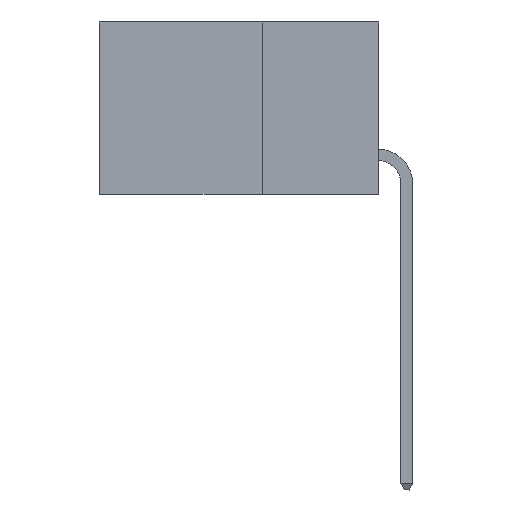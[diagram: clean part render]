
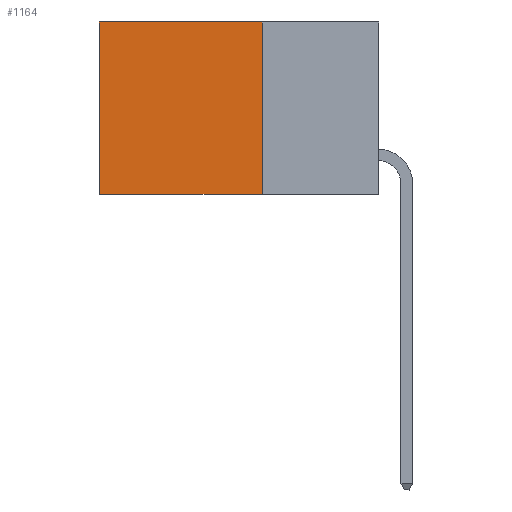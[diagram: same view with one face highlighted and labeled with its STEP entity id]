
A CAD part, left-side view. The second image highlights one B-rep face of the part: STEP entity #1164.
In plain terms, the highlighted planar face has unit normal (-1, 0, 0).
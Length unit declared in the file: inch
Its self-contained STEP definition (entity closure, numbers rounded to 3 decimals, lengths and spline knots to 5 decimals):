
#631 = VERTEX_POINT ( 'NONE', #17936 ) ;
#716 = LINE ( 'NONE', #8882, #4708 ) ;
#915 = VERTEX_POINT ( 'NONE', #16567 ) ;
#1164 = ADVANCED_FACE ( 'NONE', ( #8373 ), #3520, .F. ) ;
#2021 = VERTEX_POINT ( 'NONE', #2836 ) ;
#2396 = VECTOR ( 'NONE', #15899, 39.37008 ) ;
#2398 = VECTOR ( 'NONE', #8519, 39.37008 ) ;
#2538 = CARTESIAN_POINT ( 'NONE',  ( 0.2615, 0.25, 0. ) ) ;
#2836 = CARTESIAN_POINT ( 'NONE',  ( 0.2615, 0.25, 0. ) ) ;
#3272 = ORIENTED_EDGE ( 'NONE', *, *, #11680, .T. ) ;
#3520 = PLANE ( 'NONE',  #18665 ) ;
#3772 = EDGE_CURVE ( 'NONE', #2021, #915, #17835, .T. ) ;
#3941 = ORIENTED_EDGE ( 'NONE', *, *, #11051, .F. ) ;
#4708 = VECTOR ( 'NONE', #15148, 39.37008 ) ;
#6193 = EDGE_LOOP ( 'NONE', ( #3272, #3941, #19842, #14449 ) ) ;
#6678 = LINE ( 'NONE', #8411, #2396 ) ;
#6825 = DIRECTION ( 'NONE',  ( 1., 0., 0. ) ) ;
#8373 = FACE_OUTER_BOUND ( 'NONE', #6193, .T. ) ;
#8411 = CARTESIAN_POINT ( 'NONE',  ( 0.2615, 0.25, -0.37 ) ) ;
#8519 = DIRECTION ( 'NONE',  ( 0., 0., -1. ) ) ;
#8882 = CARTESIAN_POINT ( 'NONE',  ( 0.2615, 0.6, -0.37 ) ) ;
#8977 = VECTOR ( 'NONE', #17933, 39.37008 ) ;
#9718 = DIRECTION ( 'NONE',  ( 0., 0., -1. ) ) ;
#10059 = CARTESIAN_POINT ( 'NONE',  ( 0.2615, 0.25, -0.37 ) ) ;
#10268 = LINE ( 'NONE', #2538, #8977 ) ;
#11051 = EDGE_CURVE ( 'NONE', #915, #631, #6678, .T. ) ;
#11680 = EDGE_CURVE ( 'NONE', #17727, #631, #716, .T. ) ;
#14449 = ORIENTED_EDGE ( 'NONE', *, *, #16556, .T. ) ;
#14627 = CARTESIAN_POINT ( 'NONE',  ( 0.2615, 0.25, -0.37 ) ) ;
#14857 = CARTESIAN_POINT ( 'NONE',  ( 0.2615, 0.6, 0. ) ) ;
#15148 = DIRECTION ( 'NONE',  ( 0., 0., -1. ) ) ;
#15899 = DIRECTION ( 'NONE',  ( 0., 1., 0. ) ) ;
#16556 = EDGE_CURVE ( 'NONE', #2021, #17727, #10268, .T. ) ;
#16567 = CARTESIAN_POINT ( 'NONE',  ( 0.2615, 0.25, -0.37 ) ) ;
#17727 = VERTEX_POINT ( 'NONE', #14857 ) ;
#17835 = LINE ( 'NONE', #10059, #2398 ) ;
#17933 = DIRECTION ( 'NONE',  ( 0., 1., 0. ) ) ;
#17936 = CARTESIAN_POINT ( 'NONE',  ( 0.2615, 0.6, -0.37 ) ) ;
#18665 = AXIS2_PLACEMENT_3D ( 'NONE', #14627, #6825, #9718 ) ;
#19842 = ORIENTED_EDGE ( 'NONE', *, *, #3772, .F. ) ;
